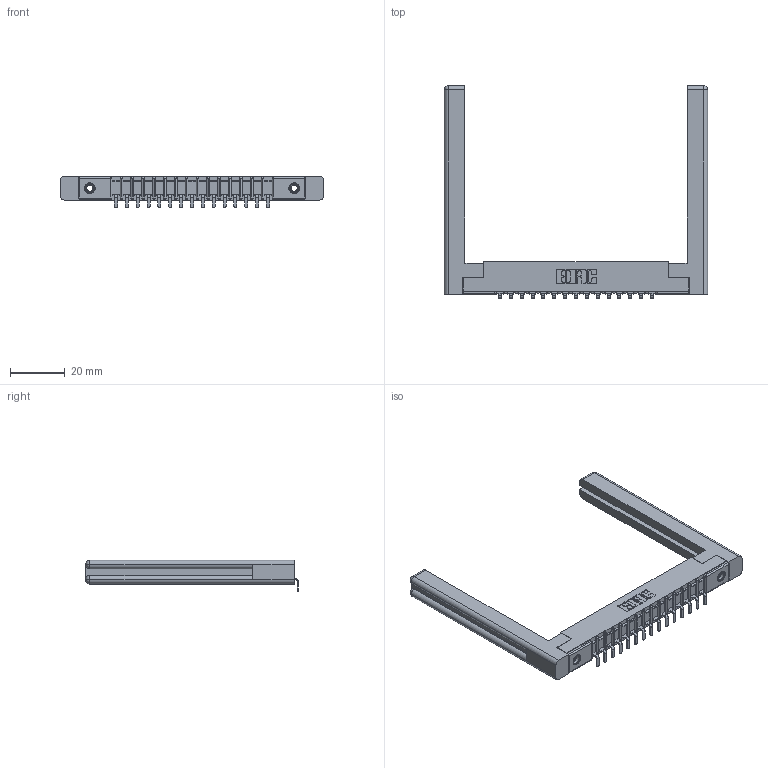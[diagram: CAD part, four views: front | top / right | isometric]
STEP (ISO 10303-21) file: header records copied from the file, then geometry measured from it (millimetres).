
FILE_DESCRIPTION (( 'STEP AP203' ), '1' );
FILE_NAME ('357-015-453-158.STEP', '2020-09-30T18:07:48', ( '' ), ( '' ), 'SwSTEP 2.0', 'SolidWorks 2020', '' );
FILE_SCHEMA (( 'CONFIG_CONTROL_DESIGN' ));
Length unit declared in the file: inch
Products named in the file (5): 307-290-002_553; 307 Part_.156 Dia Mounting Holes; 357-015-453-158; 345-250-001_345-250-001-102; 307-220-058
Assembly tree (20 placements, depth 2):
  357-015-453-158
    307 Part_.156 Dia Mounting Holes
    307-290-002_553  x15
    307-220-058  x2
    345-250-001_345-250-001-102  x2
Bounding box: 96.06 x 77.64 x 11.51 mm (x, y, z)
Volume: 14016.5 mm3; surface area: 16167.7 mm2
Topology: 20 solids, 20 shells, 1446 faces, 4337 edges, 2834 vertices
Faces by surface type: plane 859, cylinder 531, sphere 32, torus 12, cone 12
Entity records: 19675 total; most frequent: CARTESIAN_POINT 3323, ORIENTED_EDGE 3252, DIRECTION 3202, EDGE_CURVE 1626, VECTOR 1228, LINE 1228, VERTEX_POINT 1054, AXIS2_PLACEMENT_3D 987
